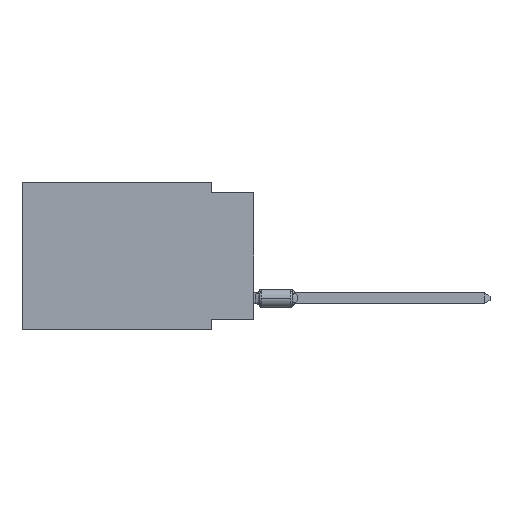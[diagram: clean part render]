
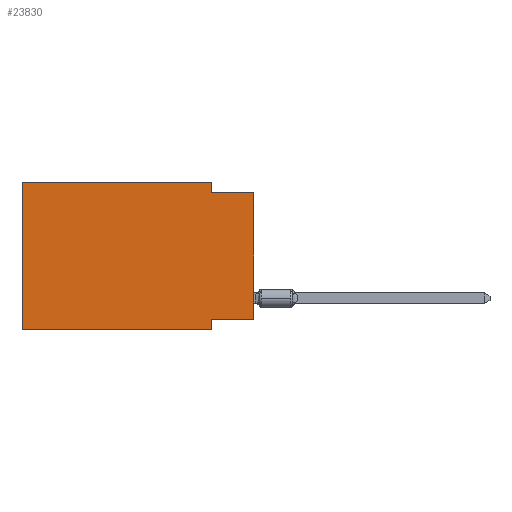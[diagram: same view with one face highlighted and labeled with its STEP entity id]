
A CAD part, left-side view. The second image highlights one B-rep face of the part: STEP entity #23830.
In plain terms, the highlighted planar face has unit normal (-1, 0, 0).
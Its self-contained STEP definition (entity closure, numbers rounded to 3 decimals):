
#208 = LINE ( 'NONE', #12744, #15718 ) ;
#589 = CARTESIAN_POINT ( 'NONE',  ( 0., 13.97, 0. ) ) ;
#809 = VERTEX_POINT ( 'NONE', #19350 ) ;
#1087 = ORIENTED_EDGE ( 'NONE', *, *, #9249, .F. ) ;
#1695 = EDGE_CURVE ( 'NONE', #21583, #15150, #2122, .T. ) ;
#2122 = LINE ( 'NONE', #19016, #16694 ) ;
#3307 = CARTESIAN_POINT ( 'NONE',  ( 0., 13.97, 0. ) ) ;
#3325 = CARTESIAN_POINT ( 'NONE',  ( 0., 2.54, -8.89 ) ) ;
#3446 = EDGE_CURVE ( 'NONE', #12707, #21583, #11254, .T. ) ;
#4400 = VECTOR ( 'NONE', #19042, 1000. ) ;
#5050 = LINE ( 'NONE', #7222, #23509 ) ;
#5090 = LINE ( 'NONE', #3307, #18063 ) ;
#5608 = LINE ( 'NONE', #14054, #17285 ) ;
#5646 = ORIENTED_EDGE ( 'NONE', *, *, #14783, .F. ) ;
#5989 = LINE ( 'NONE', #14295, #4400 ) ;
#6096 = LINE ( 'NONE', #20123, #13209 ) ;
#7222 = CARTESIAN_POINT ( 'NONE',  ( 0., 0., 0. ) ) ;
#7244 = ORIENTED_EDGE ( 'NONE', *, *, #13402, .F. ) ;
#7682 = VERTEX_POINT ( 'NONE', #13180 ) ;
#8519 = DIRECTION ( 'NONE',  ( 0., 1., 0. ) ) ;
#9249 = EDGE_CURVE ( 'NONE', #809, #9414, #5989, .T. ) ;
#9263 = ORIENTED_EDGE ( 'NONE', *, *, #21314, .T. ) ;
#9361 = CARTESIAN_POINT ( 'NONE',  ( 0., 13.97, -8.89 ) ) ;
#9414 = VERTEX_POINT ( 'NONE', #3325 ) ;
#10888 = VERTEX_POINT ( 'NONE', #9361 ) ;
#11222 = DIRECTION ( 'NONE',  ( 0., 0., 1. ) ) ;
#11254 = LINE ( 'NONE', #21600, #13275 ) ;
#12580 = FACE_OUTER_BOUND ( 'NONE', #15969, .T. ) ;
#12707 = VERTEX_POINT ( 'NONE', #13969 ) ;
#12744 = CARTESIAN_POINT ( 'NONE',  ( 0., 0., -8.255 ) ) ;
#13180 = CARTESIAN_POINT ( 'NONE',  ( 0., 0., -8.255 ) ) ;
#13209 = VECTOR ( 'NONE', #26368, 1000. ) ;
#13275 = VECTOR ( 'NONE', #21472, 1000. ) ;
#13344 = ORIENTED_EDGE ( 'NONE', *, *, #22334, .F. ) ;
#13402 = EDGE_CURVE ( 'NONE', #24623, #12707, #6096, .T. ) ;
#13969 = CARTESIAN_POINT ( 'NONE',  ( 0., 2.54, 0. ) ) ;
#14054 = CARTESIAN_POINT ( 'NONE',  ( 0., 13.97, -8.89 ) ) ;
#14295 = CARTESIAN_POINT ( 'NONE',  ( 0., 2.54, -8.89 ) ) ;
#14316 = DIRECTION ( 'NONE',  ( 0., -1., 0. ) ) ;
#14783 = EDGE_CURVE ( 'NONE', #10888, #24623, #5090, .T. ) ;
#15150 = VERTEX_POINT ( 'NONE', #25736 ) ;
#15718 = VECTOR ( 'NONE', #8519, 1000. ) ;
#15969 = EDGE_LOOP ( 'NONE', ( #9263, #16758, #17169, #7244, #5646, #20571, #1087, #13344 ) ) ;
#16487 = EDGE_CURVE ( 'NONE', #10888, #9414, #5608, .T. ) ;
#16694 = VECTOR ( 'NONE', #17620, 1000. ) ;
#16758 = ORIENTED_EDGE ( 'NONE', *, *, #1695, .F. ) ;
#17169 = ORIENTED_EDGE ( 'NONE', *, *, #3446, .F. ) ;
#17217 = DIRECTION ( 'NONE',  ( 0., 0., -1. ) ) ;
#17285 = VECTOR ( 'NONE', #14316, 1000. ) ;
#17620 = DIRECTION ( 'NONE',  ( 0., -1., 0. ) ) ;
#18063 = VECTOR ( 'NONE', #11222, 1000. ) ;
#18984 = DIRECTION ( 'NONE',  ( 1., 0., 0. ) ) ;
#19016 = CARTESIAN_POINT ( 'NONE',  ( 0., 0., -0.635 ) ) ;
#19042 = DIRECTION ( 'NONE',  ( 0., 0., -1. ) ) ;
#19252 = PLANE ( 'NONE',  #23498 ) ;
#19350 = CARTESIAN_POINT ( 'NONE',  ( 0., 2.54, -8.255 ) ) ;
#20123 = CARTESIAN_POINT ( 'NONE',  ( 0., 13.97, 0. ) ) ;
#20571 = ORIENTED_EDGE ( 'NONE', *, *, #16487, .T. ) ;
#21314 = EDGE_CURVE ( 'NONE', #7682, #15150, #5050, .T. ) ;
#21472 = DIRECTION ( 'NONE',  ( 0., 0., -1. ) ) ;
#21583 = VERTEX_POINT ( 'NONE', #24891 ) ;
#21600 = CARTESIAN_POINT ( 'NONE',  ( 0., 2.54, 0. ) ) ;
#22334 = EDGE_CURVE ( 'NONE', #7682, #809, #208, .T. ) ;
#23498 = AXIS2_PLACEMENT_3D ( 'NONE', #589, #18984, #17217 ) ;
#23509 = VECTOR ( 'NONE', #25726, 1000. ) ;
#23830 = ADVANCED_FACE ( 'NONE', ( #12580 ), #19252, .F. ) ;
#24623 = VERTEX_POINT ( 'NONE', #25533 ) ;
#24891 = CARTESIAN_POINT ( 'NONE',  ( 0., 2.54, -0.635 ) ) ;
#25533 = CARTESIAN_POINT ( 'NONE',  ( 0., 13.97, 0. ) ) ;
#25726 = DIRECTION ( 'NONE',  ( 0., 0., 1. ) ) ;
#25736 = CARTESIAN_POINT ( 'NONE',  ( 0., 0., -0.635 ) ) ;
#26368 = DIRECTION ( 'NONE',  ( 0., -1., 0. ) ) ;
